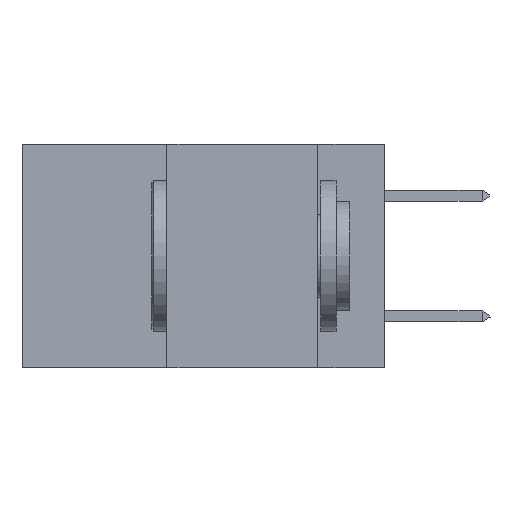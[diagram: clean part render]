
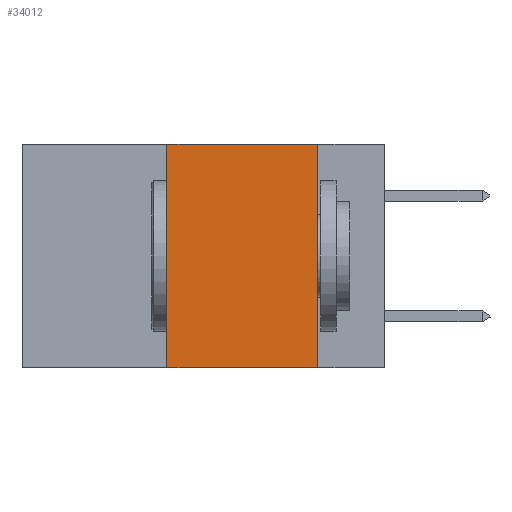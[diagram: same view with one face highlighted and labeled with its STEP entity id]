
A CAD part, left-side view. The second image highlights one B-rep face of the part: STEP entity #34012.
In plain terms, the highlighted planar face has unit normal (-1, 0, 0).
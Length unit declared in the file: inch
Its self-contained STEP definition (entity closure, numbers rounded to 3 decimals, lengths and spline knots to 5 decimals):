
#389 = AXIS2_PLACEMENT_3D ( 'NONE', #3853, #35594, #9240 ) ;
#556 = LINE ( 'NONE', #29380, #34775 ) ;
#779 = VECTOR ( 'NONE', #36642, 39.37008 ) ;
#1071 = CARTESIAN_POINT ( 'NONE',  ( 0., 0.11, 0. ) ) ;
#2517 = DIRECTION ( 'NONE',  ( 0., -1., 0. ) ) ;
#3390 = LINE ( 'NONE', #1071, #15347 ) ;
#3508 = VECTOR ( 'NONE', #2517, 39.37008 ) ;
#3808 = ORIENTED_EDGE ( 'NONE', *, *, #28066, .F. ) ;
#3853 = CARTESIAN_POINT ( 'NONE',  ( 0., 0.6, 0. ) ) ;
#6381 = DIRECTION ( 'NONE',  ( 0., -1., 0. ) ) ;
#9240 = DIRECTION ( 'NONE',  ( 0., 0., -1. ) ) ;
#10393 = VERTEX_POINT ( 'NONE', #11480 ) ;
#11480 = CARTESIAN_POINT ( 'NONE',  ( 0., 0.11, -0.37 ) ) ;
#12409 = CARTESIAN_POINT ( 'NONE',  ( 0., 0.36, 0. ) ) ;
#13833 = CARTESIAN_POINT ( 'NONE',  ( 0., 0.36, -0.37 ) ) ;
#15347 = VECTOR ( 'NONE', #21592, 39.37008 ) ;
#17315 = LINE ( 'NONE', #28060, #779 ) ;
#20625 = FACE_OUTER_BOUND ( 'NONE', #28742, .T. ) ;
#21592 = DIRECTION ( 'NONE',  ( 0., 0., -1. ) ) ;
#22562 = VERTEX_POINT ( 'NONE', #13833 ) ;
#23828 = ORIENTED_EDGE ( 'NONE', *, *, #24659, .F. ) ;
#24659 = EDGE_CURVE ( 'NONE', #22562, #37714, #17315, .T. ) ;
#24719 = ORIENTED_EDGE ( 'NONE', *, *, #34848, .T. ) ;
#26622 = EDGE_CURVE ( 'NONE', #35354, #10393, #3390, .T. ) ;
#28060 = CARTESIAN_POINT ( 'NONE',  ( 0., 0.36, 0. ) ) ;
#28066 = EDGE_CURVE ( 'NONE', #37714, #35354, #556, .T. ) ;
#28742 = EDGE_LOOP ( 'NONE', ( #29537, #3808, #23828, #24719 ) ) ;
#29380 = CARTESIAN_POINT ( 'NONE',  ( 0., 0.6, 0. ) ) ;
#29537 = ORIENTED_EDGE ( 'NONE', *, *, #26622, .F. ) ;
#30974 = LINE ( 'NONE', #37435, #3508 ) ;
#31777 = CARTESIAN_POINT ( 'NONE',  ( 0., 0.11, 0. ) ) ;
#34012 = ADVANCED_FACE ( 'NONE', ( #20625 ), #35863, .F. ) ;
#34775 = VECTOR ( 'NONE', #6381, 39.37008 ) ;
#34848 = EDGE_CURVE ( 'NONE', #22562, #10393, #30974, .T. ) ;
#35354 = VERTEX_POINT ( 'NONE', #31777 ) ;
#35594 = DIRECTION ( 'NONE',  ( 1., 0., 0. ) ) ;
#35863 = PLANE ( 'NONE',  #389 ) ;
#36642 = DIRECTION ( 'NONE',  ( 0., 0., 1. ) ) ;
#37435 = CARTESIAN_POINT ( 'NONE',  ( 0., 0.6, -0.37 ) ) ;
#37714 = VERTEX_POINT ( 'NONE', #12409 ) ;
